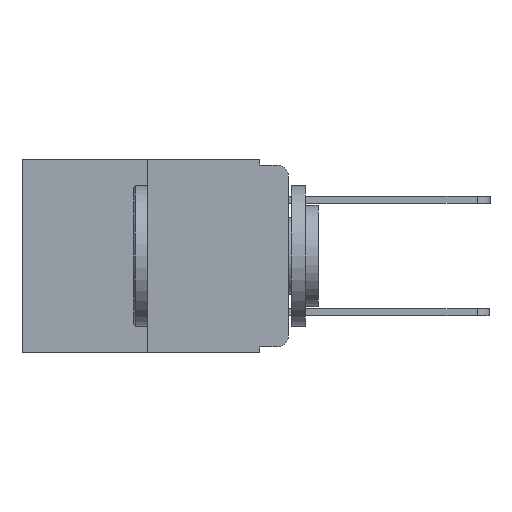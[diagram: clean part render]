
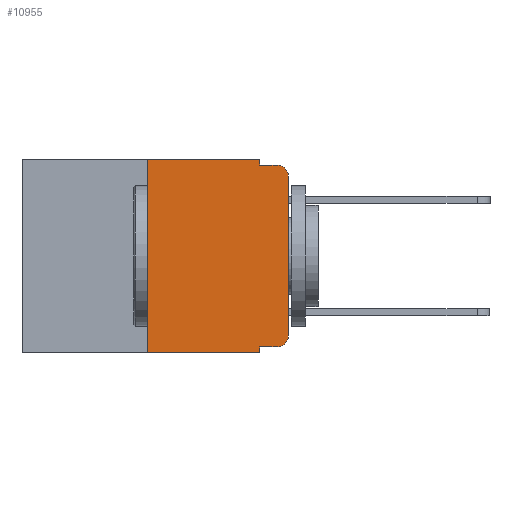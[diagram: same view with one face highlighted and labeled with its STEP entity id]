
A CAD part, left-side view. The second image highlights one B-rep face of the part: STEP entity #10955.
In plain terms, the highlighted planar face has unit normal (-1, 0, 0).
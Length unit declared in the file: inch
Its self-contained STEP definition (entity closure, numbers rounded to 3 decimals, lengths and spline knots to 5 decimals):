
#211 = CARTESIAN_POINT ( 'NONE',  ( 0., 0.051, -0.333 ) ) ;
#215 = ORIENTED_EDGE ( 'NONE', *, *, #11262, .T. ) ;
#463 = CARTESIAN_POINT ( 'NONE',  ( 0., 0., 0. ) ) ;
#944 = VERTEX_POINT ( 'NONE', #7280 ) ;
#1660 = EDGE_CURVE ( 'NONE', #5709, #944, #10606, .T. ) ;
#1790 = LINE ( 'NONE', #11105, #13726 ) ;
#1815 = VECTOR ( 'NONE', #15617, 39.37008 ) ;
#1928 = CARTESIAN_POINT ( 'NONE',  ( 0., 0.051, 0. ) ) ;
#2394 = CARTESIAN_POINT ( 'NONE',  ( 0., 0., -0.313 ) ) ;
#2607 = CARTESIAN_POINT ( 'NONE',  ( 0., 0.02, -0.03 ) ) ;
#2756 = ORIENTED_EDGE ( 'NONE', *, *, #11885, .F. ) ;
#2832 = VERTEX_POINT ( 'NONE', #16842 ) ;
#3325 = DIRECTION ( 'NONE',  ( 1., 0., 0. ) ) ;
#3535 = CARTESIAN_POINT ( 'NONE',  ( 0., 0.051, -0.01 ) ) ;
#3770 = ORIENTED_EDGE ( 'NONE', *, *, #1660, .F. ) ;
#3803 = EDGE_CURVE ( 'NONE', #2832, #13682, #6782, .T. ) ;
#4225 = DIRECTION ( 'NONE',  ( 0., 0., -1. ) ) ;
#4518 = CARTESIAN_POINT ( 'NONE',  ( 0., 0.051, -0.343 ) ) ;
#4619 = EDGE_CURVE ( 'NONE', #5709, #13045, #9874, .T. ) ;
#5679 = VECTOR ( 'NONE', #10293, 39.37008 ) ;
#5709 = VERTEX_POINT ( 'NONE', #15973 ) ;
#5735 = VECTOR ( 'NONE', #6202, 39.37008 ) ;
#5766 = CARTESIAN_POINT ( 'NONE',  ( 0., 0.02, -0.01 ) ) ;
#5782 = DIRECTION ( 'NONE',  ( -1., 0., 0. ) ) ;
#6156 = LINE ( 'NONE', #211, #1815 ) ;
#6202 = DIRECTION ( 'NONE',  ( 0., -1., 0. ) ) ;
#6392 = VECTOR ( 'NONE', #18509, 39.37008 ) ;
#6702 = CIRCLE ( 'NONE', #7933, 0.02 ) ;
#6782 = LINE ( 'NONE', #9967, #17659 ) ;
#6947 = FACE_OUTER_BOUND ( 'NONE', #14469, .T. ) ;
#7280 = CARTESIAN_POINT ( 'NONE',  ( 0., 0.25, 0. ) ) ;
#7564 = VERTEX_POINT ( 'NONE', #2394 ) ;
#7804 = CARTESIAN_POINT ( 'NONE',  ( 0., 0.051, -0.333 ) ) ;
#7823 = CARTESIAN_POINT ( 'NONE',  ( 0., 0.051, -0.01 ) ) ;
#7933 = AXIS2_PLACEMENT_3D ( 'NONE', #2607, #13475, #4225 ) ;
#8103 = CARTESIAN_POINT ( 'NONE',  ( 0., 0.473, 0. ) ) ;
#8608 = AXIS2_PLACEMENT_3D ( 'NONE', #14738, #5782, #15998 ) ;
#8857 = EDGE_CURVE ( 'NONE', #13682, #16013, #14224, .T. ) ;
#9285 = ORIENTED_EDGE ( 'NONE', *, *, #8857, .F. ) ;
#9621 = PLANE ( 'NONE',  #16498 ) ;
#9666 = VECTOR ( 'NONE', #9951, 39.37008 ) ;
#9756 = VERTEX_POINT ( 'NONE', #7804 ) ;
#9874 = LINE ( 'NONE', #13900, #16760 ) ;
#9896 = LINE ( 'NONE', #463, #5679 ) ;
#9951 = DIRECTION ( 'NONE',  ( 0., 0., -1. ) ) ;
#9967 = CARTESIAN_POINT ( 'NONE',  ( 0., 0.051, 0. ) ) ;
#10293 = DIRECTION ( 'NONE',  ( 0., 0., 1. ) ) ;
#10606 = LINE ( 'NONE', #18568, #6392 ) ;
#10803 = EDGE_CURVE ( 'NONE', #11511, #16013, #6702, .T. ) ;
#10955 = ADVANCED_FACE ( 'NONE', ( #6947 ), #9621, .F. ) ;
#11049 = EDGE_CURVE ( 'NONE', #9756, #13045, #12734, .T. ) ;
#11105 = CARTESIAN_POINT ( 'NONE',  ( 0., 0.473, 0. ) ) ;
#11162 = EDGE_CURVE ( 'NONE', #7564, #11511, #9896, .T. ) ;
#11262 = EDGE_CURVE ( 'NONE', #17685, #7564, #15585, .T. ) ;
#11511 = VERTEX_POINT ( 'NONE', #18144 ) ;
#11514 = EDGE_CURVE ( 'NONE', #9756, #17685, #6156, .T. ) ;
#11885 = EDGE_CURVE ( 'NONE', #944, #2832, #1790, .T. ) ;
#12131 = ORIENTED_EDGE ( 'NONE', *, *, #11514, .T. ) ;
#12575 = DIRECTION ( 'NONE',  ( 0., -1., 0. ) ) ;
#12734 = LINE ( 'NONE', #1928, #9666 ) ;
#12816 = ORIENTED_EDGE ( 'NONE', *, *, #10803, .T. ) ;
#12965 = DIRECTION ( 'NONE',  ( 0., 0., -1. ) ) ;
#13045 = VERTEX_POINT ( 'NONE', #4518 ) ;
#13475 = DIRECTION ( 'NONE',  ( -1., 0., 0. ) ) ;
#13682 = VERTEX_POINT ( 'NONE', #3535 ) ;
#13726 = VECTOR ( 'NONE', #12575, 39.37008 ) ;
#13900 = CARTESIAN_POINT ( 'NONE',  ( 0., 0.473, -0.343 ) ) ;
#14056 = DIRECTION ( 'NONE',  ( 0., 0., -1. ) ) ;
#14063 = ORIENTED_EDGE ( 'NONE', *, *, #3803, .F. ) ;
#14224 = LINE ( 'NONE', #7823, #5735 ) ;
#14469 = EDGE_LOOP ( 'NONE', ( #19136, #12816, #9285, #14063, #2756, #3770, #18864, #19244, #12131, #215 ) ) ;
#14738 = CARTESIAN_POINT ( 'NONE',  ( 0., 0.02, -0.313 ) ) ;
#14753 = CARTESIAN_POINT ( 'NONE',  ( 0., 0.02, -0.333 ) ) ;
#15214 = DIRECTION ( 'NONE',  ( 0., -1., 0. ) ) ;
#15585 = CIRCLE ( 'NONE', #8608, 0.02 ) ;
#15617 = DIRECTION ( 'NONE',  ( 0., -1., 0. ) ) ;
#15973 = CARTESIAN_POINT ( 'NONE',  ( 0., 0.25, -0.343 ) ) ;
#15998 = DIRECTION ( 'NONE',  ( 0., 0., -1. ) ) ;
#16013 = VERTEX_POINT ( 'NONE', #5766 ) ;
#16498 = AXIS2_PLACEMENT_3D ( 'NONE', #8103, #3325, #14056 ) ;
#16760 = VECTOR ( 'NONE', #15214, 39.37008 ) ;
#16842 = CARTESIAN_POINT ( 'NONE',  ( 0., 0.051, 0. ) ) ;
#17659 = VECTOR ( 'NONE', #12965, 39.37008 ) ;
#17685 = VERTEX_POINT ( 'NONE', #14753 ) ;
#18144 = CARTESIAN_POINT ( 'NONE',  ( 0., 0., -0.03 ) ) ;
#18509 = DIRECTION ( 'NONE',  ( 0., 0., 1. ) ) ;
#18568 = CARTESIAN_POINT ( 'NONE',  ( 0., 0.25, 0. ) ) ;
#18864 = ORIENTED_EDGE ( 'NONE', *, *, #4619, .T. ) ;
#19136 = ORIENTED_EDGE ( 'NONE', *, *, #11162, .T. ) ;
#19244 = ORIENTED_EDGE ( 'NONE', *, *, #11049, .F. ) ;
